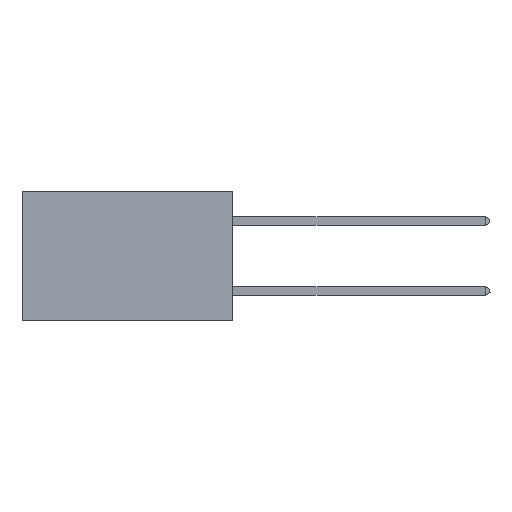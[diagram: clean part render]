
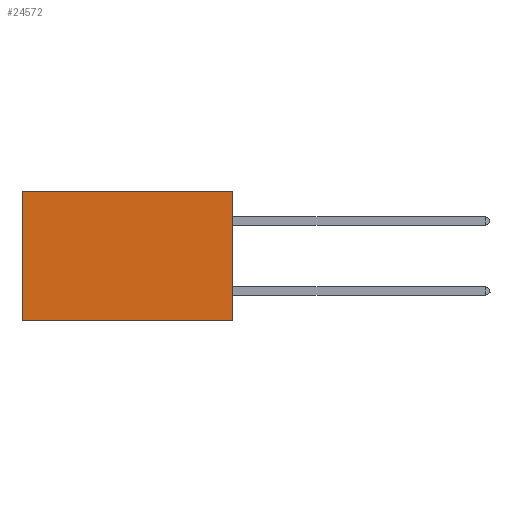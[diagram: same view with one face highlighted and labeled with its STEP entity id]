
A CAD part, left-side view. The second image highlights one B-rep face of the part: STEP entity #24572.
In plain terms, the highlighted planar face has unit normal (-1, 0, 0).
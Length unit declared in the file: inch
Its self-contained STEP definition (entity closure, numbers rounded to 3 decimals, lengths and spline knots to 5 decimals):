
#103 = CARTESIAN_POINT ( 'NONE',  ( 0.2875, 0., 0. ) ) ;
#485 = AXIS2_PLACEMENT_3D ( 'NONE', #1750, #4312, #27128 ) ;
#1750 = CARTESIAN_POINT ( 'NONE',  ( 0.2875, 0., 0. ) ) ;
#1922 = LINE ( 'NONE', #103, #24852 ) ;
#2198 = DIRECTION ( 'NONE',  ( 0., 0., -1. ) ) ;
#4312 = DIRECTION ( 'NONE',  ( 1., 0., 0. ) ) ;
#6611 = EDGE_LOOP ( 'NONE', ( #28179, #30116, #14144, #10057 ) ) ;
#7281 = VECTOR ( 'NONE', #2198, 39.37008 ) ;
#7407 = CARTESIAN_POINT ( 'NONE',  ( 0.2875, 0., 0. ) ) ;
#7672 = LINE ( 'NONE', #25173, #7281 ) ;
#8253 = CARTESIAN_POINT ( 'NONE',  ( 0.2875, 0.6, -0.37 ) ) ;
#9366 = VERTEX_POINT ( 'NONE', #8253 ) ;
#10035 = FACE_OUTER_BOUND ( 'NONE', #6611, .T. ) ;
#10057 = ORIENTED_EDGE ( 'NONE', *, *, #14781, .T. ) ;
#10697 = CARTESIAN_POINT ( 'NONE',  ( 0.2875, 0., 0. ) ) ;
#12067 = EDGE_CURVE ( 'NONE', #15939, #9366, #7672, .T. ) ;
#12778 = DIRECTION ( 'NONE',  ( 0., 0., -1. ) ) ;
#13894 = CARTESIAN_POINT ( 'NONE',  ( 0.2875, 0.6, 0. ) ) ;
#14144 = ORIENTED_EDGE ( 'NONE', *, *, #20745, .F. ) ;
#14269 = PLANE ( 'NONE',  #485 ) ;
#14561 = VERTEX_POINT ( 'NONE', #7407 ) ;
#14781 = EDGE_CURVE ( 'NONE', #14561, #15939, #31144, .T. ) ;
#15589 = LINE ( 'NONE', #18755, #19134 ) ;
#15939 = VERTEX_POINT ( 'NONE', #13894 ) ;
#18755 = CARTESIAN_POINT ( 'NONE',  ( 0.2875, 0., -0.37 ) ) ;
#19134 = VECTOR ( 'NONE', #28420, 39.37008 ) ;
#20745 = EDGE_CURVE ( 'NONE', #14561, #29957, #1922, .T. ) ;
#20929 = DIRECTION ( 'NONE',  ( 0., 1., 0. ) ) ;
#21839 = CARTESIAN_POINT ( 'NONE',  ( 0.2875, 0., -0.37 ) ) ;
#24572 = ADVANCED_FACE ( 'NONE', ( #10035 ), #14269, .F. ) ;
#24852 = VECTOR ( 'NONE', #12778, 39.37008 ) ;
#25173 = CARTESIAN_POINT ( 'NONE',  ( 0.2875, 0.6, 0. ) ) ;
#25246 = VECTOR ( 'NONE', #20929, 39.37008 ) ;
#27128 = DIRECTION ( 'NONE',  ( 0., 0., -1. ) ) ;
#28179 = ORIENTED_EDGE ( 'NONE', *, *, #12067, .T. ) ;
#28420 = DIRECTION ( 'NONE',  ( 0., 1., 0. ) ) ;
#29813 = EDGE_CURVE ( 'NONE', #29957, #9366, #15589, .T. ) ;
#29957 = VERTEX_POINT ( 'NONE', #21839 ) ;
#30116 = ORIENTED_EDGE ( 'NONE', *, *, #29813, .F. ) ;
#31144 = LINE ( 'NONE', #10697, #25246 ) ;
